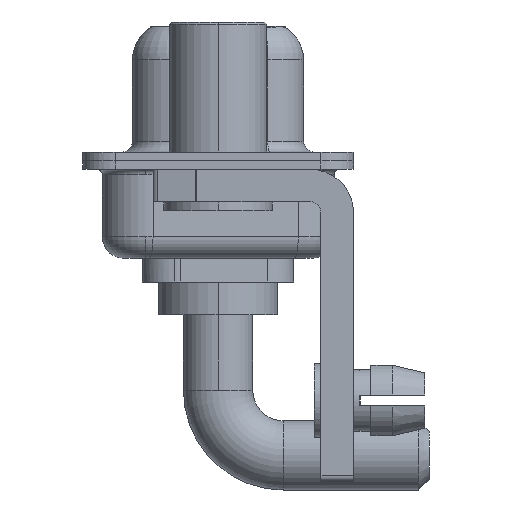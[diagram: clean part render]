
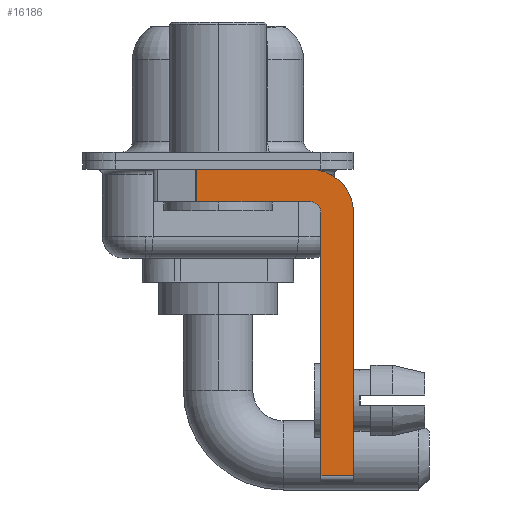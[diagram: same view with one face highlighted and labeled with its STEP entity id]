
A CAD part, left-side view. The second image highlights one B-rep face of the part: STEP entity #16186.
In plain terms, the highlighted planar face has unit normal (-1, 0, 0).
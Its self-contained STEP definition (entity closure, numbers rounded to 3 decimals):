
#3 = DIRECTION ( 'NONE',  ( 0., 0., -1. ) ) ;
#125 = VECTOR ( 'NONE', #11703, 1000. ) ;
#636 = FACE_OUTER_BOUND ( 'NONE', #1449, .T. ) ;
#695 = DIRECTION ( 'NONE',  ( 0., 0., 1. ) ) ;
#707 = ORIENTED_EDGE ( 'NONE', *, *, #16141, .T. ) ;
#736 = VERTEX_POINT ( 'NONE', #10923 ) ;
#761 = ORIENTED_EDGE ( 'NONE', *, *, #16895, .F. ) ;
#880 = EDGE_CURVE ( 'NONE', #6268, #2959, #8706, .T. ) ;
#1359 = DIRECTION ( 'NONE',  ( 0., -1., 0. ) ) ;
#1449 = EDGE_LOOP ( 'NONE', ( #7155, #707, #2016, #761, #15493, #16805, #12351, #17215 ) ) ;
#1874 = PLANE ( 'NONE',  #2697 ) ;
#2016 = ORIENTED_EDGE ( 'NONE', *, *, #10991, .F. ) ;
#2047 = CARTESIAN_POINT ( 'NONE',  ( -2.9, -4.75, -14.8 ) ) ;
#2137 = DIRECTION ( 'NONE',  ( 1., 0., 0. ) ) ;
#2491 = VECTOR ( 'NONE', #8306, 1000. ) ;
#2697 = AXIS2_PLACEMENT_3D ( 'NONE', #4607, #2137, #15503 ) ;
#2959 = VERTEX_POINT ( 'NONE', #15236 ) ;
#3050 = VECTOR ( 'NONE', #12690, 1000. ) ;
#3461 = LINE ( 'NONE', #8450, #11664 ) ;
#4217 = CARTESIAN_POINT ( 'NONE',  ( -2.9, -4.75, -14.55 ) ) ;
#4589 = CARTESIAN_POINT ( 'NONE',  ( -2.9, 0.978, -1.9 ) ) ;
#4607 = CARTESIAN_POINT ( 'NONE',  ( -2.9, -4.25, -2.4 ) ) ;
#4745 = CARTESIAN_POINT ( 'NONE',  ( -2.9, -4.25, -2.4 ) ) ;
#5305 = VERTEX_POINT ( 'NONE', #12249 ) ;
#5740 = AXIS2_PLACEMENT_3D ( 'NONE', #14961, #13374, #3 ) ;
#5777 = LINE ( 'NONE', #15017, #2491 ) ;
#5801 = DIRECTION ( 'NONE',  ( -1., 0., 0. ) ) ;
#5994 = DIRECTION ( 'NONE',  ( 0., -1., 0. ) ) ;
#6025 = VERTEX_POINT ( 'NONE', #11514 ) ;
#6268 = VERTEX_POINT ( 'NONE', #4217 ) ;
#7155 = ORIENTED_EDGE ( 'NONE', *, *, #10638, .F. ) ;
#7608 = CARTESIAN_POINT ( 'NONE',  ( -2.9, -4.75, -2.4 ) ) ;
#8061 = VERTEX_POINT ( 'NONE', #7608 ) ;
#8306 = DIRECTION ( 'NONE',  ( 0., 0., -1. ) ) ;
#8450 = CARTESIAN_POINT ( 'NONE',  ( -2.9, 0.978, -1.9 ) ) ;
#8706 = LINE ( 'NONE', #15330, #12584 ) ;
#8877 = EDGE_CURVE ( 'NONE', #6268, #8061, #17019, .T. ) ;
#9090 = LINE ( 'NONE', #9353, #14856 ) ;
#9214 = LINE ( 'NONE', #11690, #3050 ) ;
#9353 = CARTESIAN_POINT ( 'NONE',  ( -2.9, 3., -0.4 ) ) ;
#10573 = AXIS2_PLACEMENT_3D ( 'NONE', #4745, #5801, #695 ) ;
#10638 = EDGE_CURVE ( 'NONE', #17420, #5305, #9090, .T. ) ;
#10923 = CARTESIAN_POINT ( 'NONE',  ( -2.9, -4.25, -1.9 ) ) ;
#10991 = EDGE_CURVE ( 'NONE', #736, #12509, #9214, .T. ) ;
#11310 = CARTESIAN_POINT ( 'NONE',  ( -2.9, 0.978, -0.4 ) ) ;
#11514 = CARTESIAN_POINT ( 'NONE',  ( -2.9, -6.25, -2.4 ) ) ;
#11664 = VECTOR ( 'NONE', #12518, 1000. ) ;
#11690 = CARTESIAN_POINT ( 'NONE',  ( -2.9, -4.25, -1.9 ) ) ;
#11703 = DIRECTION ( 'NONE',  ( 0., 0., 1. ) ) ;
#11769 = EDGE_CURVE ( 'NONE', #6025, #2959, #5777, .T. ) ;
#12249 = CARTESIAN_POINT ( 'NONE',  ( -2.9, -4.25, -0.4 ) ) ;
#12351 = ORIENTED_EDGE ( 'NONE', *, *, #11769, .F. ) ;
#12509 = VERTEX_POINT ( 'NONE', #4589 ) ;
#12518 = DIRECTION ( 'NONE',  ( 0., 0., -1. ) ) ;
#12584 = VECTOR ( 'NONE', #5994, 1000. ) ;
#12690 = DIRECTION ( 'NONE',  ( 0., 1., 0. ) ) ;
#13374 = DIRECTION ( 'NONE',  ( 1., 0., 0. ) ) ;
#14227 = CIRCLE ( 'NONE', #10573, 0.5 ) ;
#14448 = CIRCLE ( 'NONE', #5740, 2. ) ;
#14856 = VECTOR ( 'NONE', #1359, 1000. ) ;
#14948 = EDGE_CURVE ( 'NONE', #5305, #6025, #14448, .T. ) ;
#14961 = CARTESIAN_POINT ( 'NONE',  ( -2.9, -4.25, -2.4 ) ) ;
#15017 = CARTESIAN_POINT ( 'NONE',  ( -2.9, -6.25, -2.4 ) ) ;
#15236 = CARTESIAN_POINT ( 'NONE',  ( -2.9, -6.25, -14.55 ) ) ;
#15330 = CARTESIAN_POINT ( 'NONE',  ( -2.9, -4.25, -14.55 ) ) ;
#15493 = ORIENTED_EDGE ( 'NONE', *, *, #8877, .F. ) ;
#15503 = DIRECTION ( 'NONE',  ( 0., 0., -1. ) ) ;
#16141 = EDGE_CURVE ( 'NONE', #17420, #12509, #3461, .T. ) ;
#16186 = ADVANCED_FACE ( 'NONE', ( #636 ), #1874, .F. ) ;
#16805 = ORIENTED_EDGE ( 'NONE', *, *, #880, .T. ) ;
#16895 = EDGE_CURVE ( 'NONE', #8061, #736, #14227, .T. ) ;
#17019 = LINE ( 'NONE', #2047, #125 ) ;
#17215 = ORIENTED_EDGE ( 'NONE', *, *, #14948, .F. ) ;
#17420 = VERTEX_POINT ( 'NONE', #11310 ) ;
